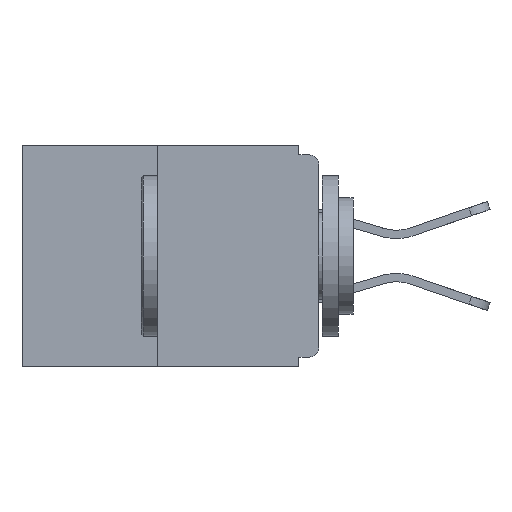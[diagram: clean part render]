
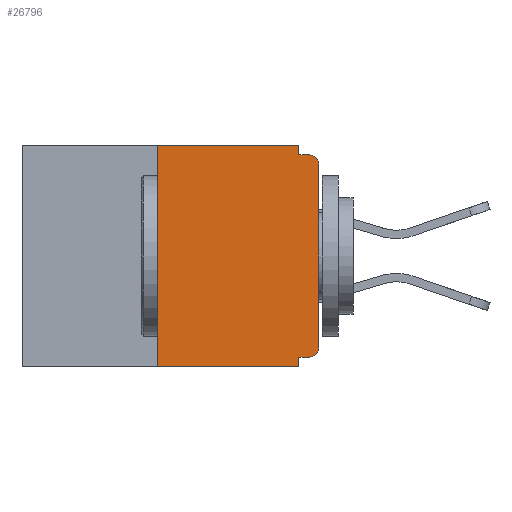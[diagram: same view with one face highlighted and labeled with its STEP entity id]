
A CAD part, left-side view. The second image highlights one B-rep face of the part: STEP entity #26796.
In plain terms, the highlighted planar face has unit normal (-1, 0, 0).
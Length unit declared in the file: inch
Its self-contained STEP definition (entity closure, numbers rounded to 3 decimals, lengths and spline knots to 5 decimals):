
#1139 = ORIENTED_EDGE ( 'NONE', *, *, #13338, .T. ) ;
#1153 = EDGE_CURVE ( 'NONE', #23230, #29370, #3925, .T. ) ;
#1329 = LINE ( 'NONE', #27346, #21884 ) ;
#1347 = VERTEX_POINT ( 'NONE', #21688 ) ;
#1508 = VERTEX_POINT ( 'NONE', #14474 ) ;
#1835 = CARTESIAN_POINT ( 'NONE',  ( 0., 0.46, 0. ) ) ;
#2266 = EDGE_CURVE ( 'NONE', #28141, #1508, #1329, .T. ) ;
#2843 = DIRECTION ( 'NONE',  ( 0., 0., -1. ) ) ;
#2897 = DIRECTION ( 'NONE',  ( 0., 0., 1. ) ) ;
#3485 = LINE ( 'NONE', #17313, #7162 ) ;
#3925 = CIRCLE ( 'NONE', #15643, 0.015 ) ;
#4232 = PLANE ( 'NONE',  #10145 ) ;
#4279 = CARTESIAN_POINT ( 'NONE',  ( 0., 0.46, 0. ) ) ;
#4532 = VECTOR ( 'NONE', #27413, 39.37008 ) ;
#4921 = ORIENTED_EDGE ( 'NONE', *, *, #7400, .T. ) ;
#5814 = VECTOR ( 'NONE', #26868, 39.37008 ) ;
#5829 = CARTESIAN_POINT ( 'NONE',  ( 0., 0.015, -0.328 ) ) ;
#6029 = DIRECTION ( 'NONE',  ( 0., 0., -1. ) ) ;
#6238 = DIRECTION ( 'NONE',  ( 0., -1., 0. ) ) ;
#6478 = DIRECTION ( 'NONE',  ( 1., 0., 0. ) ) ;
#6578 = DIRECTION ( 'NONE',  ( 0., 0., -1. ) ) ;
#6707 = ORIENTED_EDGE ( 'NONE', *, *, #2266, .F. ) ;
#6722 = CIRCLE ( 'NONE', #28484, 0.015 ) ;
#6942 = CARTESIAN_POINT ( 'NONE',  ( 0., 0., -0.328 ) ) ;
#7162 = VECTOR ( 'NONE', #6029, 39.37008 ) ;
#7212 = ORIENTED_EDGE ( 'NONE', *, *, #23719, .F. ) ;
#7362 = CARTESIAN_POINT ( 'NONE',  ( 0., 0., -0.03 ) ) ;
#7400 = EDGE_CURVE ( 'NONE', #29763, #19386, #6722, .T. ) ;
#8012 = CARTESIAN_POINT ( 'NONE',  ( 0., 0.25, 0. ) ) ;
#8232 = EDGE_CURVE ( 'NONE', #14075, #28141, #11708, .T. ) ;
#9985 = EDGE_CURVE ( 'NONE', #22985, #14075, #24596, .T. ) ;
#10114 = DIRECTION ( 'NONE',  ( -1., 0., 0. ) ) ;
#10145 = AXIS2_PLACEMENT_3D ( 'NONE', #1835, #6478, #6578 ) ;
#10820 = CARTESIAN_POINT ( 'NONE',  ( 0., 0.25, -0.343 ) ) ;
#11217 = DIRECTION ( 'NONE',  ( 0., 0., -1. ) ) ;
#11708 = LINE ( 'NONE', #4279, #13876 ) ;
#11778 = DIRECTION ( 'NONE',  ( 0., -1., 0. ) ) ;
#12087 = CARTESIAN_POINT ( 'NONE',  ( 0., 0., 0. ) ) ;
#13006 = FACE_OUTER_BOUND ( 'NONE', #25003, .T. ) ;
#13168 = CARTESIAN_POINT ( 'NONE',  ( 0., 0., -0.313 ) ) ;
#13338 = EDGE_CURVE ( 'NONE', #19386, #23230, #13451, .T. ) ;
#13451 = LINE ( 'NONE', #12087, #18833 ) ;
#13876 = VECTOR ( 'NONE', #15896, 39.37008 ) ;
#14075 = VERTEX_POINT ( 'NONE', #8012 ) ;
#14474 = CARTESIAN_POINT ( 'NONE',  ( 0., 0.031, -0.015 ) ) ;
#14539 = CARTESIAN_POINT ( 'NONE',  ( 0., 0.015, -0.03 ) ) ;
#15643 = AXIS2_PLACEMENT_3D ( 'NONE', #14539, #10114, #2843 ) ;
#15805 = ORIENTED_EDGE ( 'NONE', *, *, #9985, .F. ) ;
#15896 = DIRECTION ( 'NONE',  ( 0., -1., 0. ) ) ;
#16258 = CARTESIAN_POINT ( 'NONE',  ( 0., 0.031, 0. ) ) ;
#16946 = ORIENTED_EDGE ( 'NONE', *, *, #27601, .F. ) ;
#17313 = CARTESIAN_POINT ( 'NONE',  ( 0., 0.031, -0.343 ) ) ;
#17991 = ORIENTED_EDGE ( 'NONE', *, *, #18700, .T. ) ;
#18428 = ORIENTED_EDGE ( 'NONE', *, *, #8232, .F. ) ;
#18693 = VECTOR ( 'NONE', #11778, 39.37008 ) ;
#18700 = EDGE_CURVE ( 'NONE', #22985, #1347, #28173, .T. ) ;
#18833 = VECTOR ( 'NONE', #2897, 39.37008 ) ;
#19386 = VERTEX_POINT ( 'NONE', #13168 ) ;
#19803 = LINE ( 'NONE', #25602, #18693 ) ;
#21223 = DIRECTION ( 'NONE',  ( -1., 0., 0. ) ) ;
#21688 = CARTESIAN_POINT ( 'NONE',  ( 0., 0.031, -0.343 ) ) ;
#21884 = VECTOR ( 'NONE', #11217, 39.37008 ) ;
#22518 = CARTESIAN_POINT ( 'NONE',  ( 0., 0.031, -0.328 ) ) ;
#22702 = ORIENTED_EDGE ( 'NONE', *, *, #28322, .F. ) ;
#22985 = VERTEX_POINT ( 'NONE', #10820 ) ;
#23230 = VERTEX_POINT ( 'NONE', #7362 ) ;
#23575 = DIRECTION ( 'NONE',  ( 0., 0., -1. ) ) ;
#23719 = EDGE_CURVE ( 'NONE', #29763, #24858, #24758, .T. ) ;
#24265 = CARTESIAN_POINT ( 'NONE',  ( 0., 0.25, 0. ) ) ;
#24596 = LINE ( 'NONE', #24265, #5814 ) ;
#24758 = LINE ( 'NONE', #6942, #4532 ) ;
#24815 = CARTESIAN_POINT ( 'NONE',  ( 0., 0.46, -0.343 ) ) ;
#24858 = VERTEX_POINT ( 'NONE', #22518 ) ;
#25003 = EDGE_LOOP ( 'NONE', ( #18428, #15805, #17991, #22702, #7212, #4921, #1139, #25155, #16946, #6707 ) ) ;
#25155 = ORIENTED_EDGE ( 'NONE', *, *, #1153, .T. ) ;
#25602 = CARTESIAN_POINT ( 'NONE',  ( 0., 0., -0.015 ) ) ;
#26796 = ADVANCED_FACE ( 'NONE', ( #13006 ), #4232, .F. ) ;
#26868 = DIRECTION ( 'NONE',  ( 0., 0., 1. ) ) ;
#27346 = CARTESIAN_POINT ( 'NONE',  ( 0., 0.031, 0. ) ) ;
#27413 = DIRECTION ( 'NONE',  ( 0., 1., 0. ) ) ;
#27601 = EDGE_CURVE ( 'NONE', #1508, #29370, #19803, .T. ) ;
#27991 = CARTESIAN_POINT ( 'NONE',  ( 0., 0.015, -0.313 ) ) ;
#28020 = CARTESIAN_POINT ( 'NONE',  ( 0., 0.015, -0.015 ) ) ;
#28141 = VERTEX_POINT ( 'NONE', #16258 ) ;
#28173 = LINE ( 'NONE', #24815, #28902 ) ;
#28322 = EDGE_CURVE ( 'NONE', #24858, #1347, #3485, .T. ) ;
#28484 = AXIS2_PLACEMENT_3D ( 'NONE', #27991, #21223, #23575 ) ;
#28902 = VECTOR ( 'NONE', #6238, 39.37008 ) ;
#29370 = VERTEX_POINT ( 'NONE', #28020 ) ;
#29763 = VERTEX_POINT ( 'NONE', #5829 ) ;
